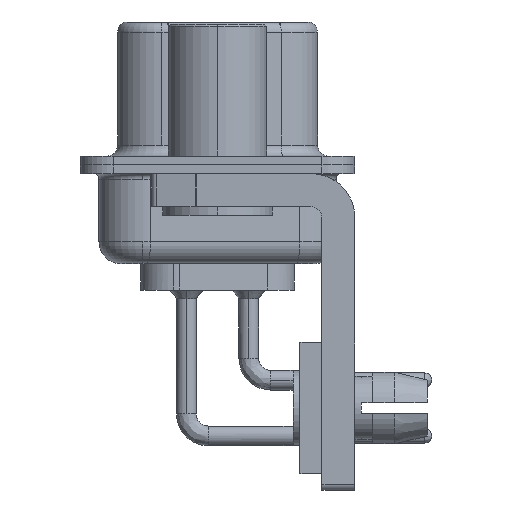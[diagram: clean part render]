
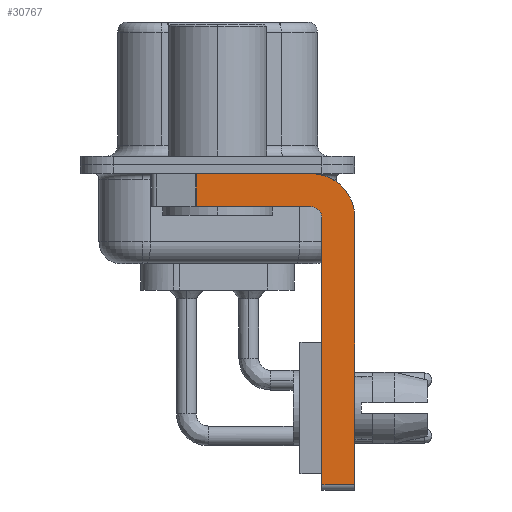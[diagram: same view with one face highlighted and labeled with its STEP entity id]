
A CAD part, left-side view. The second image highlights one B-rep face of the part: STEP entity #30767.
In plain terms, the highlighted planar face has unit normal (-1, 0, 0).
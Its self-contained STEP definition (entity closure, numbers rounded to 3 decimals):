
#689 = CARTESIAN_POINT ( 'NONE',  ( -2.9, -6.25, -14.55 ) ) ;
#1546 = LINE ( 'NONE', #34036, #23604 ) ;
#2609 = CARTESIAN_POINT ( 'NONE',  ( -2.9, -6.25, -2.4 ) ) ;
#2814 = DIRECTION ( 'NONE',  ( 0., -1., 0. ) ) ;
#3966 = EDGE_CURVE ( 'NONE', #12525, #11827, #15950, .T. ) ;
#4487 = CARTESIAN_POINT ( 'NONE',  ( -2.9, 0.978, -1.9 ) ) ;
#4595 = VECTOR ( 'NONE', #2814, 1000. ) ;
#6645 = CARTESIAN_POINT ( 'NONE',  ( -2.9, -4.75, -14.55 ) ) ;
#7294 = CARTESIAN_POINT ( 'NONE',  ( -2.9, -4.25, -1.9 ) ) ;
#7492 = AXIS2_PLACEMENT_3D ( 'NONE', #8580, #28465, #11437 ) ;
#7595 = EDGE_CURVE ( 'NONE', #11827, #31385, #11423, .T. ) ;
#8002 = ORIENTED_EDGE ( 'NONE', *, *, #17846, .F. ) ;
#8336 = EDGE_LOOP ( 'NONE', ( #25455, #9971, #23870, #18931, #13138, #23546, #8002, #18558 ) ) ;
#8580 = CARTESIAN_POINT ( 'NONE',  ( -2.9, -4.25, -2.4 ) ) ;
#9226 = LINE ( 'NONE', #30949, #15026 ) ;
#9971 = ORIENTED_EDGE ( 'NONE', *, *, #34414, .T. ) ;
#10193 = LINE ( 'NONE', #2609, #31062 ) ;
#10817 = PLANE ( 'NONE',  #31055 ) ;
#11423 = LINE ( 'NONE', #7294, #18124 ) ;
#11437 = DIRECTION ( 'NONE',  ( 0., 0., -1. ) ) ;
#11827 = VERTEX_POINT ( 'NONE', #36736 ) ;
#12525 = VERTEX_POINT ( 'NONE', #25769 ) ;
#13138 = ORIENTED_EDGE ( 'NONE', *, *, #22740, .F. ) ;
#13191 = LINE ( 'NONE', #31287, #4595 ) ;
#13274 = VECTOR ( 'NONE', #26453, 1000. ) ;
#13713 = DIRECTION ( 'NONE',  ( 0., 0., -1. ) ) ;
#15012 = CARTESIAN_POINT ( 'NONE',  ( -2.9, 3., -0.4 ) ) ;
#15026 = VECTOR ( 'NONE', #28238, 1000. ) ;
#15950 = CIRCLE ( 'NONE', #30556, 0.5 ) ;
#16974 = DIRECTION ( 'NONE',  ( 0., 0., -1. ) ) ;
#17103 = CARTESIAN_POINT ( 'NONE',  ( -2.9, 0.978, -0.4 ) ) ;
#17846 = EDGE_CURVE ( 'NONE', #27208, #31188, #10193, .T. ) ;
#18124 = VECTOR ( 'NONE', #21533, 1000. ) ;
#18558 = ORIENTED_EDGE ( 'NONE', *, *, #30894, .F. ) ;
#18931 = ORIENTED_EDGE ( 'NONE', *, *, #3966, .F. ) ;
#19644 = VERTEX_POINT ( 'NONE', #17103 ) ;
#19947 = DIRECTION ( 'NONE',  ( 0., 0., 1. ) ) ;
#20826 = LINE ( 'NONE', #15012, #13274 ) ;
#20978 = CARTESIAN_POINT ( 'NONE',  ( -2.9, -4.25, -0.4 ) ) ;
#21354 = FACE_OUTER_BOUND ( 'NONE', #8336, .T. ) ;
#21533 = DIRECTION ( 'NONE',  ( 0., 1., 0. ) ) ;
#22318 = DIRECTION ( 'NONE',  ( 0., 0., 1. ) ) ;
#22551 = DIRECTION ( 'NONE',  ( -1., 0., 0. ) ) ;
#22688 = CARTESIAN_POINT ( 'NONE',  ( -2.9, -4.25, -2.4 ) ) ;
#22740 = EDGE_CURVE ( 'NONE', #26326, #12525, #1546, .T. ) ;
#23546 = ORIENTED_EDGE ( 'NONE', *, *, #24969, .T. ) ;
#23604 = VECTOR ( 'NONE', #19947, 1000. ) ;
#23870 = ORIENTED_EDGE ( 'NONE', *, *, #7595, .F. ) ;
#24969 = EDGE_CURVE ( 'NONE', #26326, #31188, #13191, .T. ) ;
#25455 = ORIENTED_EDGE ( 'NONE', *, *, #33970, .F. ) ;
#25769 = CARTESIAN_POINT ( 'NONE',  ( -2.9, -4.75, -2.4 ) ) ;
#26326 = VERTEX_POINT ( 'NONE', #6645 ) ;
#26453 = DIRECTION ( 'NONE',  ( 0., -1., 0. ) ) ;
#27208 = VERTEX_POINT ( 'NONE', #32449 ) ;
#28238 = DIRECTION ( 'NONE',  ( 0., 0., -1. ) ) ;
#28465 = DIRECTION ( 'NONE',  ( 1., 0., 0. ) ) ;
#29906 = VERTEX_POINT ( 'NONE', #20978 ) ;
#30556 = AXIS2_PLACEMENT_3D ( 'NONE', #22688, #22551, #22318 ) ;
#30684 = DIRECTION ( 'NONE',  ( 1., 0., 0. ) ) ;
#30767 = ADVANCED_FACE ( 'NONE', ( #21354 ), #10817, .F. ) ;
#30894 = EDGE_CURVE ( 'NONE', #29906, #27208, #31955, .T. ) ;
#30949 = CARTESIAN_POINT ( 'NONE',  ( -2.9, 0.978, -1.9 ) ) ;
#31055 = AXIS2_PLACEMENT_3D ( 'NONE', #36212, #30684, #13713 ) ;
#31062 = VECTOR ( 'NONE', #16974, 1000. ) ;
#31188 = VERTEX_POINT ( 'NONE', #689 ) ;
#31287 = CARTESIAN_POINT ( 'NONE',  ( -2.9, -4.25, -14.55 ) ) ;
#31385 = VERTEX_POINT ( 'NONE', #4487 ) ;
#31955 = CIRCLE ( 'NONE', #7492, 2. ) ;
#32449 = CARTESIAN_POINT ( 'NONE',  ( -2.9, -6.25, -2.4 ) ) ;
#33970 = EDGE_CURVE ( 'NONE', #19644, #29906, #20826, .T. ) ;
#34036 = CARTESIAN_POINT ( 'NONE',  ( -2.9, -4.75, -14.8 ) ) ;
#34414 = EDGE_CURVE ( 'NONE', #19644, #31385, #9226, .T. ) ;
#36212 = CARTESIAN_POINT ( 'NONE',  ( -2.9, -4.25, -2.4 ) ) ;
#36736 = CARTESIAN_POINT ( 'NONE',  ( -2.9, -4.25, -1.9 ) ) ;
